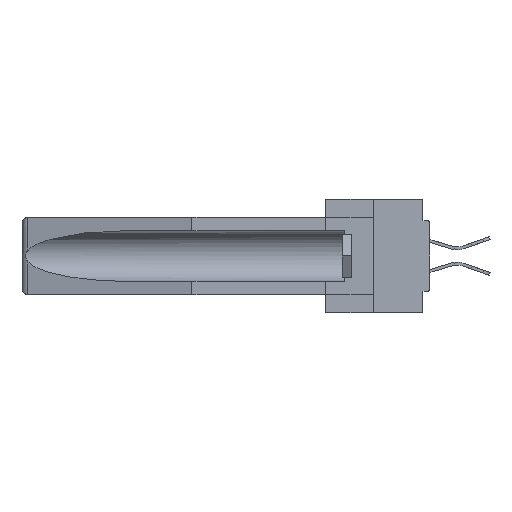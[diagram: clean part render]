
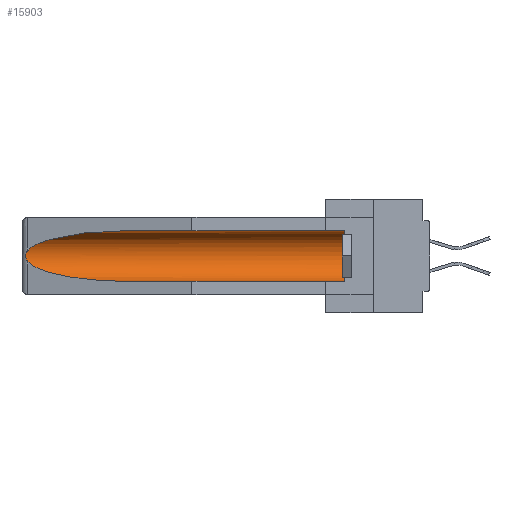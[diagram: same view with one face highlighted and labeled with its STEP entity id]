
A CAD part, left-side view. The second image highlights one B-rep face of the part: STEP entity #15903.
In plain terms, the highlighted cylindrical face has radius 2.857 mm (diameter 5.715 mm), a partial arc.
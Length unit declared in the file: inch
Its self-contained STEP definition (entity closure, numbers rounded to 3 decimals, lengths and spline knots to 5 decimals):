
#232 = VECTOR ( 'NONE', #27489, 39.37008 ) ;
#499 = ORIENTED_EDGE ( 'NONE', *, *, #21364, .T. ) ;
#570 = VERTEX_POINT ( 'NONE', #35628 ) ;
#1089 = ORIENTED_EDGE ( 'NONE', *, *, #20210, .T. ) ;
#1099 =( BOUNDED_CURVE ( )  B_SPLINE_CURVE ( 3, ( #3740, #9609, #9353, #35212 ),
 .UNSPECIFIED., .F., .F. ) 
 B_SPLINE_CURVE_WITH_KNOTS ( ( 4, 4 ),
 ( 4.71239, 6.08839 ),
 .UNSPECIFIED. ) 
 CURVE ( )  GEOMETRIC_REPRESENTATION_ITEM ( )  RATIONAL_B_SPLINE_CURVE ( ( 1., 0.848, 0.848, 1. ) ) 
 REPRESENTATION_ITEM ( '' )  );
#1781 = CARTESIAN_POINT ( 'NONE',  ( 0.155, 0.126, -0.1715 ) ) ;
#3740 = CARTESIAN_POINT ( 'NONE',  ( 0.155, 1.07973, -0.059 ) ) ;
#3817 = AXIS2_PLACEMENT_3D ( 'NONE', #11012, #11246, #25133 ) ;
#3835 =( BOUNDED_CURVE ( )  B_SPLINE_CURVE ( 3, ( #34417, #20576, #23470, #31931 ),
 .UNSPECIFIED., .F., .F. ) 
 B_SPLINE_CURVE_WITH_KNOTS ( ( 4, 4 ),
 ( 0.1948, 1.5708 ),
 .UNSPECIFIED. ) 
 CURVE ( )  GEOMETRIC_REPRESENTATION_ITEM ( )  RATIONAL_B_SPLINE_CURVE ( ( 1., 0.848, 0.848, 1. ) ) 
 REPRESENTATION_ITEM ( '' )  );
#4069 = EDGE_LOOP ( 'NONE', ( #21445, #15827, #499, #32248, #1089, #21235 ) ) ;
#5202 = VERTEX_POINT ( 'NONE', #27537 ) ;
#5672 = VECTOR ( 'NONE', #9986, 39.37008 ) ;
#6658 = CARTESIAN_POINT ( 'NONE',  ( 0.2675, 1.53308, -0.16763 ) ) ;
#7015 = LINE ( 'NONE', #35845, #5672 ) ;
#7805 = LINE ( 'NONE', #20122, #232 ) ;
#9287 = CARTESIAN_POINT ( 'NONE',  ( 0.155, 0.126, -0.059 ) ) ;
#9353 = CARTESIAN_POINT ( 'NONE',  ( 0.25451, 1.48313, -0.09465 ) ) ;
#9609 = CARTESIAN_POINT ( 'NONE',  ( 0.21114, 1.30732, -0.059 ) ) ;
#9986 = DIRECTION ( 'NONE',  ( 0., 1., 0. ) ) ;
#10521 = CARTESIAN_POINT ( 'NONE',  ( 0.155, 1.07973, -0.284 ) ) ;
#11012 = CARTESIAN_POINT ( 'NONE',  ( 0.155, -0.30754, -0.1715 ) ) ;
#11246 = DIRECTION ( 'NONE',  ( 0., 1., 0. ) ) ;
#11863 = CARTESIAN_POINT ( 'NONE',  ( 0.155, 0.126, -0.284 ) ) ;
#11921 = CARTESIAN_POINT ( 'NONE',  ( 0.26537, 1.52718, -0.14972 ) ) ;
#13716 = AXIS2_PLACEMENT_3D ( 'NONE', #1781, #29894, #30017 ) ;
#13840 = FACE_OUTER_BOUND ( 'NONE', #4069, .T. ) ;
#15827 = ORIENTED_EDGE ( 'NONE', *, *, #33459, .T. ) ;
#15903 = ADVANCED_FACE ( 'NONE', ( #13840 ), #17835, .F. ) ;
#17657 = CARTESIAN_POINT ( 'NONE',  ( 0.26597, 1.52961, -0.15275 ) ) ;
#17835 = CYLINDRICAL_SURFACE ( 'NONE', #3817, 0.1125 ) ;
#18021 = CARTESIAN_POINT ( 'NONE',  ( 0.26537, 1.52718, -0.19328 ) ) ;
#18497 = EDGE_CURVE ( 'NONE', #23451, #570, #1099, .T. ) ;
#19104 = VERTEX_POINT ( 'NONE', #10521 ) ;
#20122 = CARTESIAN_POINT ( 'NONE',  ( 0.155, -0.30754, -0.059 ) ) ;
#20210 = EDGE_CURVE ( 'NONE', #32467, #33424, #28320, .T. ) ;
#20414 = CARTESIAN_POINT ( 'NONE',  ( 0.2673, 1.53269, -0.17917 ) ) ;
#20544 = CARTESIAN_POINT ( 'NONE',  ( 0.26655, 1.53094, -0.18657 ) ) ;
#20576 = CARTESIAN_POINT ( 'NONE',  ( 0.25451, 1.48313, -0.24835 ) ) ;
#21235 = ORIENTED_EDGE ( 'NONE', *, *, #22687, .T. ) ;
#21364 = EDGE_CURVE ( 'NONE', #5202, #19104, #3835, .T. ) ;
#21445 = ORIENTED_EDGE ( 'NONE', *, *, #18497, .T. ) ;
#22378 = CARTESIAN_POINT ( 'NONE',  ( 0.155, 1.07973, -0.059 ) ) ;
#22687 = EDGE_CURVE ( 'NONE', #33424, #23451, #7805, .T. ) ;
#23451 = VERTEX_POINT ( 'NONE', #22378 ) ;
#23470 = CARTESIAN_POINT ( 'NONE',  ( 0.21114, 1.30732, -0.284 ) ) ;
#23670 = CARTESIAN_POINT ( 'NONE',  ( 0.26654, 1.53092, -0.15636 ) ) ;
#25133 = DIRECTION ( 'NONE',  ( 0., 0., 1. ) ) ;
#26313 = CARTESIAN_POINT ( 'NONE',  ( 0.26597, 1.5296, -0.19026 ) ) ;
#27489 = DIRECTION ( 'NONE',  ( 0., 1., 0. ) ) ;
#27537 = CARTESIAN_POINT ( 'NONE',  ( 0.26537, 1.52718, -0.19328 ) ) ;
#28320 = CIRCLE ( 'NONE', #13716, 0.1125 ) ;
#29894 = DIRECTION ( 'NONE',  ( 0., -1., 0. ) ) ;
#30017 = DIRECTION ( 'NONE',  ( 0., 0., 1. ) ) ;
#31894 = CARTESIAN_POINT ( 'NONE',  ( 0.2673, 1.5327, -0.16383 ) ) ;
#31931 = CARTESIAN_POINT ( 'NONE',  ( 0.155, 1.07973, -0.284 ) ) ;
#32248 = ORIENTED_EDGE ( 'NONE', *, *, #35358, .F. ) ;
#32467 = VERTEX_POINT ( 'NONE', #11863 ) ;
#33424 = VERTEX_POINT ( 'NONE', #9287 ) ;
#33459 = EDGE_CURVE ( 'NONE', #570, #5202, #34267, .T. ) ;
#34267 = B_SPLINE_CURVE_WITH_KNOTS ( 'NONE', 3,
 ( #11921, #17657, #23670, #31894, #6658, #35019, #20414, #20544, #26313, #18021 ),
 .UNSPECIFIED., .F., .F.,
 ( 4, 2, 2, 2, 4 ),
 ( 0., 0.00029, 0.00058, 0.00087, 0.00117 ),
 .UNSPECIFIED. ) ;
#34417 = CARTESIAN_POINT ( 'NONE',  ( 0.26537, 1.52718, -0.19328 ) ) ;
#35019 = CARTESIAN_POINT ( 'NONE',  ( 0.2675, 1.53308, -0.17534 ) ) ;
#35212 = CARTESIAN_POINT ( 'NONE',  ( 0.26537, 1.52718, -0.14972 ) ) ;
#35358 = EDGE_CURVE ( 'NONE', #32467, #19104, #7015, .T. ) ;
#35628 = CARTESIAN_POINT ( 'NONE',  ( 0.26537, 1.52718, -0.14972 ) ) ;
#35845 = CARTESIAN_POINT ( 'NONE',  ( 0.155, -0.30754, -0.284 ) ) ;
